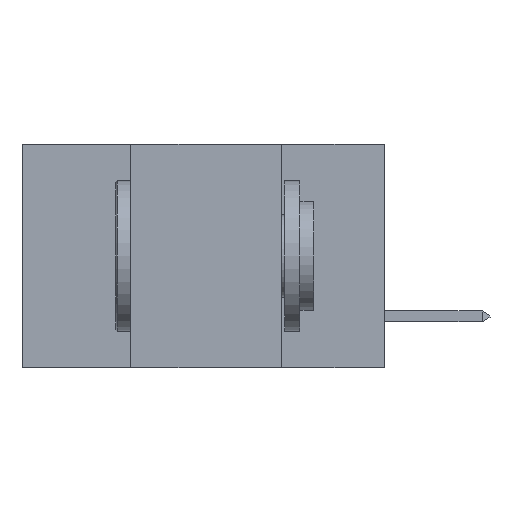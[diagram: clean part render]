
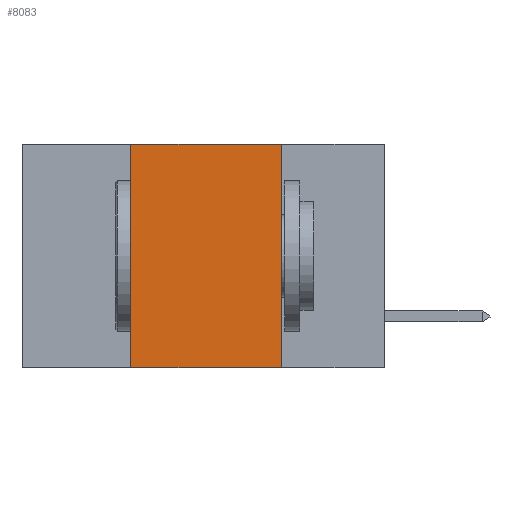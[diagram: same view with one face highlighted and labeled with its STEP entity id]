
A CAD part, left-side view. The second image highlights one B-rep face of the part: STEP entity #8083.
In plain terms, the highlighted planar face has unit normal (-1, 0, 0).
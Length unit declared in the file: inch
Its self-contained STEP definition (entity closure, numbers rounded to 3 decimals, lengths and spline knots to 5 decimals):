
#571 = LINE ( 'NONE', #13220, #12779 ) ;
#1420 = VERTEX_POINT ( 'NONE', #3183 ) ;
#1630 = VERTEX_POINT ( 'NONE', #7272 ) ;
#3183 = CARTESIAN_POINT ( 'NONE',  ( 0., 0.17, 0. ) ) ;
#5349 = DIRECTION ( 'NONE',  ( 0., -1., 0. ) ) ;
#5553 = FACE_OUTER_BOUND ( 'NONE', #27678, .T. ) ;
#6679 = VERTEX_POINT ( 'NONE', #25158 ) ;
#6974 = EDGE_CURVE ( 'NONE', #1420, #6679, #26356, .T. ) ;
#7272 = CARTESIAN_POINT ( 'NONE',  ( 0., 0.42, 0. ) ) ;
#8083 = ADVANCED_FACE ( 'NONE', ( #5553 ), #18635, .F. ) ;
#9063 = ORIENTED_EDGE ( 'NONE', *, *, #27438, .T. ) ;
#9519 = EDGE_CURVE ( 'NONE', #1630, #1420, #11557, .T. ) ;
#10824 = DIRECTION ( 'NONE',  ( 1., 0., 0. ) ) ;
#11557 = LINE ( 'NONE', #29569, #24647 ) ;
#12482 = VECTOR ( 'NONE', #26366, 39.37008 ) ;
#12779 = VECTOR ( 'NONE', #21123, 39.37008 ) ;
#13044 = LINE ( 'NONE', #15719, #32227 ) ;
#13220 = CARTESIAN_POINT ( 'NONE',  ( 0., 0.42, 0. ) ) ;
#13370 = CARTESIAN_POINT ( 'NONE',  ( 0., 0.17, 0. ) ) ;
#13964 = DIRECTION ( 'NONE',  ( 0., -1., 0. ) ) ;
#14764 = ORIENTED_EDGE ( 'NONE', *, *, #9519, .F. ) ;
#15719 = CARTESIAN_POINT ( 'NONE',  ( 0., 0.6, -0.37 ) ) ;
#18635 = PLANE ( 'NONE',  #28160 ) ;
#20841 = VERTEX_POINT ( 'NONE', #24692 ) ;
#21123 = DIRECTION ( 'NONE',  ( 0., 0., 1. ) ) ;
#22561 = ORIENTED_EDGE ( 'NONE', *, *, #33342, .F. ) ;
#23876 = CARTESIAN_POINT ( 'NONE',  ( 0., 0.6, 0. ) ) ;
#24647 = VECTOR ( 'NONE', #13964, 39.37008 ) ;
#24692 = CARTESIAN_POINT ( 'NONE',  ( 0., 0.42, -0.37 ) ) ;
#25158 = CARTESIAN_POINT ( 'NONE',  ( 0., 0.17, -0.37 ) ) ;
#26356 = LINE ( 'NONE', #13370, #12482 ) ;
#26366 = DIRECTION ( 'NONE',  ( 0., 0., -1. ) ) ;
#26558 = ORIENTED_EDGE ( 'NONE', *, *, #6974, .F. ) ;
#27438 = EDGE_CURVE ( 'NONE', #20841, #6679, #13044, .T. ) ;
#27678 = EDGE_LOOP ( 'NONE', ( #26558, #14764, #22561, #9063 ) ) ;
#28160 = AXIS2_PLACEMENT_3D ( 'NONE', #23876, #10824, #29096 ) ;
#29096 = DIRECTION ( 'NONE',  ( 0., 0., -1. ) ) ;
#29569 = CARTESIAN_POINT ( 'NONE',  ( 0., 0.6, 0. ) ) ;
#32227 = VECTOR ( 'NONE', #5349, 39.37008 ) ;
#33342 = EDGE_CURVE ( 'NONE', #20841, #1630, #571, .T. ) ;
